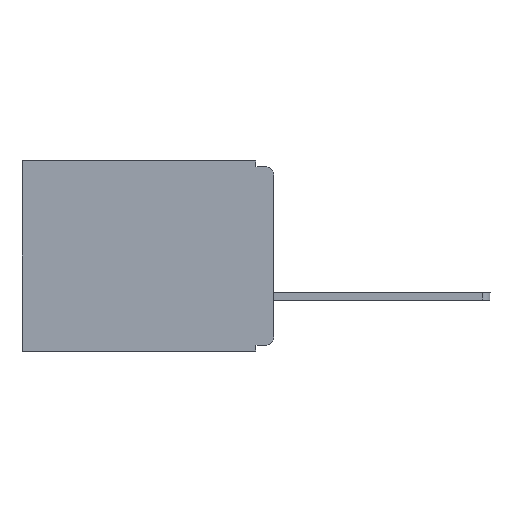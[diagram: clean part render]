
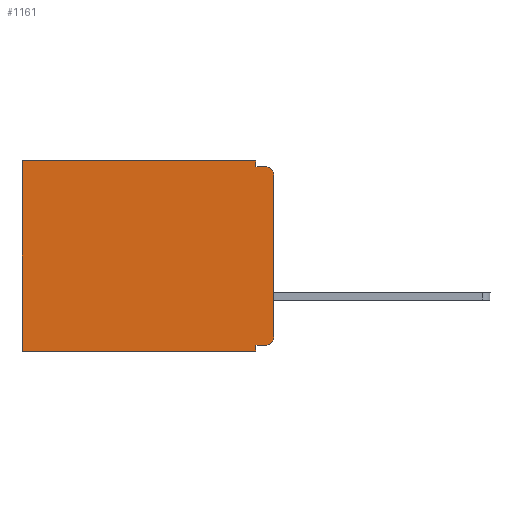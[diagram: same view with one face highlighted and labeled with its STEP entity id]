
A CAD part, left-side view. The second image highlights one B-rep face of the part: STEP entity #1161.
In plain terms, the highlighted planar face has unit normal (-1, 0, 0).
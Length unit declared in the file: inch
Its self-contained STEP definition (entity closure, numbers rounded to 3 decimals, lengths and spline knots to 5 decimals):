
#172 = AXIS2_PLACEMENT_3D ( 'NONE', #1234, #2024, #10019 ) ;
#378 = DIRECTION ( 'NONE',  ( 0., 0., -1. ) ) ;
#497 = VECTOR ( 'NONE', #2032, 39.37008 ) ;
#540 = VECTOR ( 'NONE', #5718, 39.37008 ) ;
#630 = CARTESIAN_POINT ( 'NONE',  ( 0.3, 0., -0.025 ) ) ;
#743 = ORIENTED_EDGE ( 'NONE', *, *, #5456, .T. ) ;
#787 = EDGE_CURVE ( 'NONE', #1580, #1230, #2240, .T. ) ;
#935 = VERTEX_POINT ( 'NONE', #11386 ) ;
#964 = CIRCLE ( 'NONE', #7492, 0.015 ) ;
#1005 = CARTESIAN_POINT ( 'NONE',  ( 0.3, 0., -0.305 ) ) ;
#1065 = CARTESIAN_POINT ( 'NONE',  ( 0.3, 0.031, -0.33 ) ) ;
#1161 = ADVANCED_FACE ( 'NONE', ( #6441 ), #10738, .F. ) ;
#1230 = VERTEX_POINT ( 'NONE', #1005 ) ;
#1234 = CARTESIAN_POINT ( 'NONE',  ( 0.3, 0.015, -0.025 ) ) ;
#1333 = CARTESIAN_POINT ( 'NONE',  ( 0.3, 0.437, 0. ) ) ;
#1478 = DIRECTION ( 'NONE',  ( 0., 1., 0. ) ) ;
#1489 = DIRECTION ( 'NONE',  ( 0., 0., -1. ) ) ;
#1547 = VERTEX_POINT ( 'NONE', #6058 ) ;
#1580 = VERTEX_POINT ( 'NONE', #630 ) ;
#1842 = LINE ( 'NONE', #8691, #8881 ) ;
#1961 = VECTOR ( 'NONE', #9133, 39.37008 ) ;
#2024 = DIRECTION ( 'NONE',  ( -1., 0., 0. ) ) ;
#2032 = DIRECTION ( 'NONE',  ( 0., 0., -1. ) ) ;
#2084 = LINE ( 'NONE', #4267, #7856 ) ;
#2240 = LINE ( 'NONE', #5798, #540 ) ;
#2687 = CARTESIAN_POINT ( 'NONE',  ( 0.3, 0., -0.33 ) ) ;
#3008 = VERTEX_POINT ( 'NONE', #3376 ) ;
#3048 = CARTESIAN_POINT ( 'NONE',  ( 0.3, 0.437, -0.33 ) ) ;
#3161 = LINE ( 'NONE', #1065, #497 ) ;
#3206 = VERTEX_POINT ( 'NONE', #5647 ) ;
#3227 = ORIENTED_EDGE ( 'NONE', *, *, #5505, .T. ) ;
#3291 = EDGE_CURVE ( 'NONE', #11421, #10890, #4601, .T. ) ;
#3293 = CARTESIAN_POINT ( 'NONE',  ( 0.3, 0.031, 0. ) ) ;
#3376 = CARTESIAN_POINT ( 'NONE',  ( 0.3, 0.015, -0.01 ) ) ;
#3660 = DIRECTION ( 'NONE',  ( 0., 0., -1. ) ) ;
#4012 = CARTESIAN_POINT ( 'NONE',  ( 0.3, 0.437, -0.33 ) ) ;
#4041 = EDGE_CURVE ( 'NONE', #10270, #1230, #964, .T. ) ;
#4236 = DIRECTION ( 'NONE',  ( 0., -1., 0. ) ) ;
#4267 = CARTESIAN_POINT ( 'NONE',  ( 0.3, 0., -0.01 ) ) ;
#4333 = DIRECTION ( 'NONE',  ( -1., 0., 0. ) ) ;
#4601 = LINE ( 'NONE', #3048, #7163 ) ;
#4657 = CARTESIAN_POINT ( 'NONE',  ( 0.3, 0., 0. ) ) ;
#4783 = CARTESIAN_POINT ( 'NONE',  ( 0.3, 0., -0.32 ) ) ;
#5264 = ORIENTED_EDGE ( 'NONE', *, *, #7215, .F. ) ;
#5456 = EDGE_CURVE ( 'NONE', #1580, #3008, #8581, .T. ) ;
#5505 = EDGE_CURVE ( 'NONE', #5645, #11421, #9269, .T. ) ;
#5513 = LINE ( 'NONE', #4783, #8059 ) ;
#5645 = VERTEX_POINT ( 'NONE', #3293 ) ;
#5647 = CARTESIAN_POINT ( 'NONE',  ( 0.3, 0.031, -0.32 ) ) ;
#5700 = DIRECTION ( 'NONE',  ( 0., 1., 0. ) ) ;
#5718 = DIRECTION ( 'NONE',  ( 0., 0., -1. ) ) ;
#5798 = CARTESIAN_POINT ( 'NONE',  ( 0.3, 0., -0.33 ) ) ;
#6055 = CARTESIAN_POINT ( 'NONE',  ( 0.3, 0.015, -0.305 ) ) ;
#6058 = CARTESIAN_POINT ( 'NONE',  ( 0.3, 0.031, -0.01 ) ) ;
#6277 = ORIENTED_EDGE ( 'NONE', *, *, #3291, .T. ) ;
#6306 = DIRECTION ( 'NONE',  ( 1., 0., 0. ) ) ;
#6441 = FACE_OUTER_BOUND ( 'NONE', #8257, .T. ) ;
#6921 = ORIENTED_EDGE ( 'NONE', *, *, #9227, .F. ) ;
#7039 = AXIS2_PLACEMENT_3D ( 'NONE', #2687, #6306, #3660 ) ;
#7146 = ORIENTED_EDGE ( 'NONE', *, *, #4041, .T. ) ;
#7163 = VECTOR ( 'NONE', #378, 39.37008 ) ;
#7215 = EDGE_CURVE ( 'NONE', #1547, #3008, #2084, .T. ) ;
#7492 = AXIS2_PLACEMENT_3D ( 'NONE', #6055, #4333, #9734 ) ;
#7827 = EDGE_CURVE ( 'NONE', #3206, #935, #3161, .T. ) ;
#7856 = VECTOR ( 'NONE', #4236, 39.37008 ) ;
#8059 = VECTOR ( 'NONE', #5700, 39.37008 ) ;
#8216 = ORIENTED_EDGE ( 'NONE', *, *, #10994, .F. ) ;
#8257 = EDGE_LOOP ( 'NONE', ( #8968, #743, #5264, #8216, #3227, #6277, #11394, #9382, #6921, #7146 ) ) ;
#8581 = CIRCLE ( 'NONE', #172, 0.015 ) ;
#8644 = CARTESIAN_POINT ( 'NONE',  ( 0.3, 0., -0.33 ) ) ;
#8691 = CARTESIAN_POINT ( 'NONE',  ( 0.3, 0.031, 0. ) ) ;
#8881 = VECTOR ( 'NONE', #1489, 39.37008 ) ;
#8968 = ORIENTED_EDGE ( 'NONE', *, *, #787, .F. ) ;
#9133 = DIRECTION ( 'NONE',  ( 0., 1., 0. ) ) ;
#9227 = EDGE_CURVE ( 'NONE', #10270, #3206, #5513, .T. ) ;
#9269 = LINE ( 'NONE', #4657, #1961 ) ;
#9382 = ORIENTED_EDGE ( 'NONE', *, *, #7827, .F. ) ;
#9734 = DIRECTION ( 'NONE',  ( 0., 0., -1. ) ) ;
#10019 = DIRECTION ( 'NONE',  ( 0., 0., -1. ) ) ;
#10101 = LINE ( 'NONE', #8644, #11451 ) ;
#10270 = VERTEX_POINT ( 'NONE', #10510 ) ;
#10510 = CARTESIAN_POINT ( 'NONE',  ( 0.3, 0.015, -0.32 ) ) ;
#10738 = PLANE ( 'NONE',  #7039 ) ;
#10890 = VERTEX_POINT ( 'NONE', #4012 ) ;
#10994 = EDGE_CURVE ( 'NONE', #5645, #1547, #1842, .T. ) ;
#11386 = CARTESIAN_POINT ( 'NONE',  ( 0.3, 0.031, -0.33 ) ) ;
#11394 = ORIENTED_EDGE ( 'NONE', *, *, #11418, .F. ) ;
#11418 = EDGE_CURVE ( 'NONE', #935, #10890, #10101, .T. ) ;
#11421 = VERTEX_POINT ( 'NONE', #1333 ) ;
#11451 = VECTOR ( 'NONE', #1478, 39.37008 ) ;
